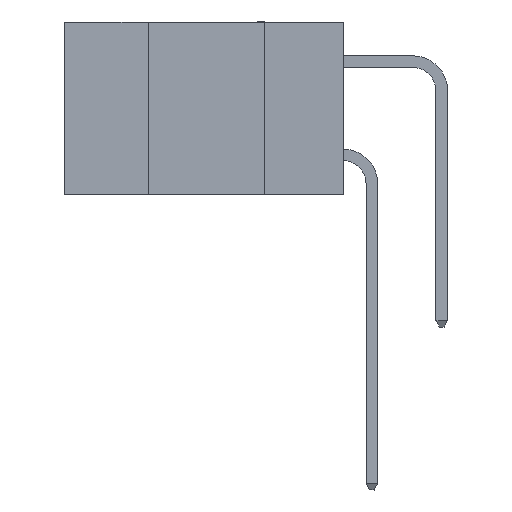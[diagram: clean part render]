
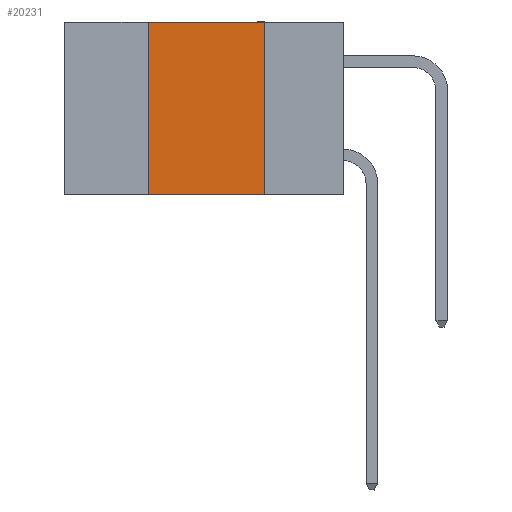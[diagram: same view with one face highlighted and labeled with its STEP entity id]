
A CAD part, left-side view. The second image highlights one B-rep face of the part: STEP entity #20231.
In plain terms, the highlighted planar face has unit normal (-1, 0, 0).
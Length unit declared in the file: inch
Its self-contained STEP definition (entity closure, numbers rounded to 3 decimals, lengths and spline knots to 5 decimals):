
#39 = CARTESIAN_POINT ( 'NONE',  ( 0., 0.42, 0. ) ) ;
#42 = PLANE ( 'NONE',  #2597 ) ;
#59 = VERTEX_POINT ( 'NONE', #39 ) ;
#700 = CARTESIAN_POINT ( 'NONE',  ( 0., 0.6, 0. ) ) ;
#831 = EDGE_CURVE ( 'NONE', #59, #20244, #21247, .T. ) ;
#990 = CARTESIAN_POINT ( 'NONE',  ( 0., 0.42, -0.37 ) ) ;
#1063 = ORIENTED_EDGE ( 'NONE', *, *, #27003, .T. ) ;
#1637 = DIRECTION ( 'NONE',  ( 0., 0., 1. ) ) ;
#2461 = VECTOR ( 'NONE', #13826, 39.37008 ) ;
#2597 = AXIS2_PLACEMENT_3D ( 'NONE', #7228, #23667, #9561 ) ;
#3259 = LINE ( 'NONE', #13432, #27545 ) ;
#3372 = DIRECTION ( 'NONE',  ( 0., -1., 0. ) ) ;
#4116 = EDGE_LOOP ( 'NONE', ( #8469, #9925, #16168, #1063 ) ) ;
#4249 = CARTESIAN_POINT ( 'NONE',  ( 0., 0.6, -0.37 ) ) ;
#5961 = EDGE_CURVE ( 'NONE', #10384, #59, #3259, .T. ) ;
#7228 = CARTESIAN_POINT ( 'NONE',  ( 0., 0.6, 0. ) ) ;
#8348 = DIRECTION ( 'NONE',  ( 0., 0., -1. ) ) ;
#8469 = ORIENTED_EDGE ( 'NONE', *, *, #18493, .F. ) ;
#9561 = DIRECTION ( 'NONE',  ( 0., 0., -1. ) ) ;
#9925 = ORIENTED_EDGE ( 'NONE', *, *, #831, .F. ) ;
#10384 = VERTEX_POINT ( 'NONE', #990 ) ;
#13432 = CARTESIAN_POINT ( 'NONE',  ( 0., 0.42, 0. ) ) ;
#13826 = DIRECTION ( 'NONE',  ( 0., -1., 0. ) ) ;
#14322 = CARTESIAN_POINT ( 'NONE',  ( 0., 0.17, 0. ) ) ;
#16168 = ORIENTED_EDGE ( 'NONE', *, *, #5961, .F. ) ;
#18493 = EDGE_CURVE ( 'NONE', #20244, #29086, #30449, .T. ) ;
#19735 = VECTOR ( 'NONE', #3372, 39.37008 ) ;
#19741 = FACE_OUTER_BOUND ( 'NONE', #4116, .T. ) ;
#20231 = ADVANCED_FACE ( 'NONE', ( #19741 ), #42, .F. ) ;
#20244 = VERTEX_POINT ( 'NONE', #14322 ) ;
#21247 = LINE ( 'NONE', #700, #19735 ) ;
#23464 = VECTOR ( 'NONE', #8348, 39.37008 ) ;
#23503 = CARTESIAN_POINT ( 'NONE',  ( 0., 0.17, -0.37 ) ) ;
#23667 = DIRECTION ( 'NONE',  ( 1., 0., 0. ) ) ;
#27003 = EDGE_CURVE ( 'NONE', #10384, #29086, #28208, .T. ) ;
#27545 = VECTOR ( 'NONE', #1637, 39.37008 ) ;
#28208 = LINE ( 'NONE', #4249, #2461 ) ;
#29086 = VERTEX_POINT ( 'NONE', #23503 ) ;
#29396 = CARTESIAN_POINT ( 'NONE',  ( 0., 0.17, 0. ) ) ;
#30449 = LINE ( 'NONE', #29396, #23464 ) ;
